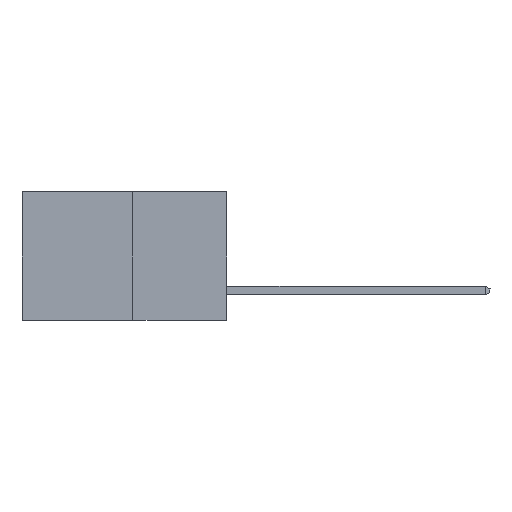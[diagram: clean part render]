
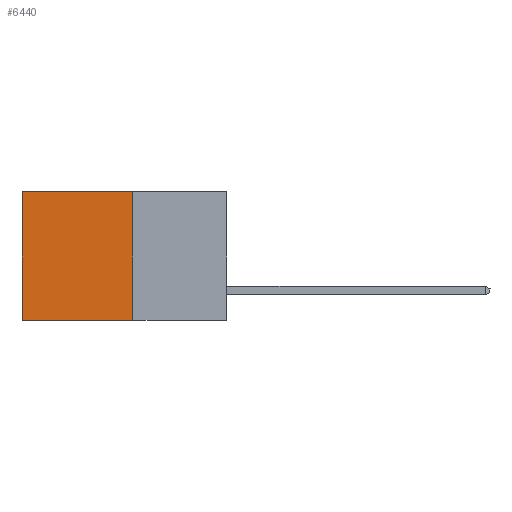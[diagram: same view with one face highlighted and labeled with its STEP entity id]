
A CAD part, left-side view. The second image highlights one B-rep face of the part: STEP entity #6440.
In plain terms, the highlighted planar face has unit normal (-1, 0, 0).
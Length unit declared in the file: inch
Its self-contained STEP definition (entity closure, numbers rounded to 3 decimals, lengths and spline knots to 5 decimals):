
#217 = LINE ( 'NONE', #7815, #9513 ) ;
#304 = VERTEX_POINT ( 'NONE', #3866 ) ;
#352 = VERTEX_POINT ( 'NONE', #5824 ) ;
#495 = ORIENTED_EDGE ( 'NONE', *, *, #8264, .F. ) ;
#1363 = AXIS2_PLACEMENT_3D ( 'NONE', #9498, #9687, #10961 ) ;
#1566 = LINE ( 'NONE', #5377, #10581 ) ;
#2675 = EDGE_CURVE ( 'NONE', #4061, #352, #10793, .T. ) ;
#2826 = ORIENTED_EDGE ( 'NONE', *, *, #9679, .T. ) ;
#3080 = VECTOR ( 'NONE', #8581, 39.37008 ) ;
#3327 = PLANE ( 'NONE',  #1363 ) ;
#3866 = CARTESIAN_POINT ( 'NONE',  ( 0.277, 0.59, -0.37 ) ) ;
#4061 = VERTEX_POINT ( 'NONE', #10301 ) ;
#5186 = CARTESIAN_POINT ( 'NONE',  ( 0.277, 0.27, 0. ) ) ;
#5377 = CARTESIAN_POINT ( 'NONE',  ( 0.277, 0.27, -0.37 ) ) ;
#5565 = ORIENTED_EDGE ( 'NONE', *, *, #2675, .T. ) ;
#5604 = EDGE_CURVE ( 'NONE', #7674, #304, #8069, .T. ) ;
#5824 = CARTESIAN_POINT ( 'NONE',  ( 0.277, 0.59, 0. ) ) ;
#6440 = ADVANCED_FACE ( 'NONE', ( #9060 ), #3327, .F. ) ;
#6466 = VECTOR ( 'NONE', #7725, 39.37008 ) ;
#7047 = CARTESIAN_POINT ( 'NONE',  ( 0.277, 0.27, -0.37 ) ) ;
#7236 = EDGE_LOOP ( 'NONE', ( #2826, #7598, #495, #5565 ) ) ;
#7598 = ORIENTED_EDGE ( 'NONE', *, *, #5604, .F. ) ;
#7674 = VERTEX_POINT ( 'NONE', #9547 ) ;
#7725 = DIRECTION ( 'NONE',  ( 0., 1., 0. ) ) ;
#7815 = CARTESIAN_POINT ( 'NONE',  ( 0.277, 0.59, -0.37 ) ) ;
#7975 = DIRECTION ( 'NONE',  ( 0., 0., -1. ) ) ;
#8069 = LINE ( 'NONE', #7047, #3080 ) ;
#8264 = EDGE_CURVE ( 'NONE', #4061, #7674, #1566, .T. ) ;
#8581 = DIRECTION ( 'NONE',  ( 0., 1., 0. ) ) ;
#9060 = FACE_OUTER_BOUND ( 'NONE', #7236, .T. ) ;
#9498 = CARTESIAN_POINT ( 'NONE',  ( 0.277, 0.27, -0.37 ) ) ;
#9513 = VECTOR ( 'NONE', #11009, 39.37008 ) ;
#9547 = CARTESIAN_POINT ( 'NONE',  ( 0.277, 0.27, -0.37 ) ) ;
#9679 = EDGE_CURVE ( 'NONE', #352, #304, #217, .T. ) ;
#9687 = DIRECTION ( 'NONE',  ( 1., 0., 0. ) ) ;
#10301 = CARTESIAN_POINT ( 'NONE',  ( 0.277, 0.27, 0. ) ) ;
#10581 = VECTOR ( 'NONE', #7975, 39.37008 ) ;
#10793 = LINE ( 'NONE', #5186, #6466 ) ;
#10961 = DIRECTION ( 'NONE',  ( 0., 0., -1. ) ) ;
#11009 = DIRECTION ( 'NONE',  ( 0., 0., -1. ) ) ;
